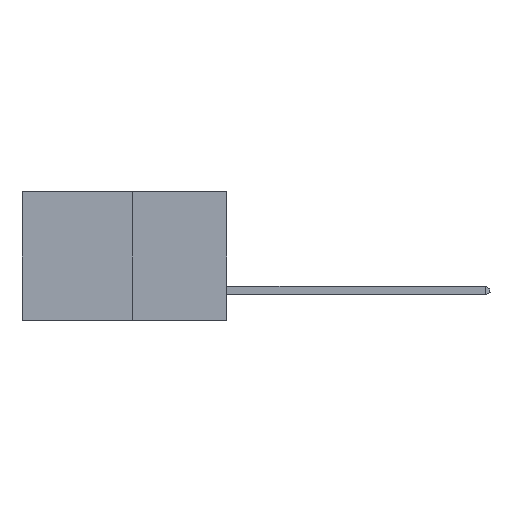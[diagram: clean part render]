
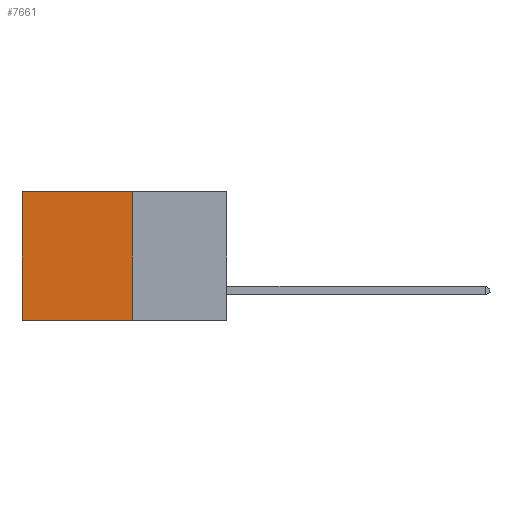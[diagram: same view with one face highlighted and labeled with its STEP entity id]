
A CAD part, left-side view. The second image highlights one B-rep face of the part: STEP entity #7661.
In plain terms, the highlighted planar face has unit normal (-1, 0, 0).
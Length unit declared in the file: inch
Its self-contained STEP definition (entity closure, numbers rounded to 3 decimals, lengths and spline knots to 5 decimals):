
#938 = EDGE_LOOP ( 'NONE', ( #30658, #7178, #3249, #1567 ) ) ;
#1088 = VERTEX_POINT ( 'NONE', #22789 ) ;
#1567 = ORIENTED_EDGE ( 'NONE', *, *, #18640, .T. ) ;
#1786 = DIRECTION ( 'NONE',  ( 0., 0., -1. ) ) ;
#2138 = DIRECTION ( 'NONE',  ( 0., 1., 0. ) ) ;
#2320 = DIRECTION ( 'NONE',  ( 0., 0., -1. ) ) ;
#3249 = ORIENTED_EDGE ( 'NONE', *, *, #10928, .F. ) ;
#3741 = CARTESIAN_POINT ( 'NONE',  ( 0.277, 0.27, -0.37 ) ) ;
#3883 = DIRECTION ( 'NONE',  ( 1., 0., 0. ) ) ;
#7178 = ORIENTED_EDGE ( 'NONE', *, *, #29767, .F. ) ;
#7661 = ADVANCED_FACE ( 'NONE', ( #13336 ), #24814, .F. ) ;
#8039 = CARTESIAN_POINT ( 'NONE',  ( 0.277, 0.59, 0. ) ) ;
#10627 = VERTEX_POINT ( 'NONE', #16747 ) ;
#10928 = EDGE_CURVE ( 'NONE', #10627, #14963, #24257, .T. ) ;
#13336 = FACE_OUTER_BOUND ( 'NONE', #938, .T. ) ;
#14853 = VECTOR ( 'NONE', #2138, 39.37008 ) ;
#14963 = VERTEX_POINT ( 'NONE', #3741 ) ;
#15121 = AXIS2_PLACEMENT_3D ( 'NONE', #19726, #3883, #22331 ) ;
#16747 = CARTESIAN_POINT ( 'NONE',  ( 0.277, 0.27, 0. ) ) ;
#17963 = CARTESIAN_POINT ( 'NONE',  ( 0.277, 0.27, -0.37 ) ) ;
#18640 = EDGE_CURVE ( 'NONE', #10627, #21871, #26075, .T. ) ;
#18955 = VECTOR ( 'NONE', #2320, 39.37008 ) ;
#19156 = VECTOR ( 'NONE', #22991, 39.37008 ) ;
#19726 = CARTESIAN_POINT ( 'NONE',  ( 0.277, 0.27, -0.37 ) ) ;
#20398 = CARTESIAN_POINT ( 'NONE',  ( 0.277, 0.27, -0.37 ) ) ;
#21871 = VERTEX_POINT ( 'NONE', #8039 ) ;
#22331 = DIRECTION ( 'NONE',  ( 0., 0., -1. ) ) ;
#22789 = CARTESIAN_POINT ( 'NONE',  ( 0.277, 0.59, -0.37 ) ) ;
#22866 = EDGE_CURVE ( 'NONE', #21871, #1088, #32841, .T. ) ;
#22881 = CARTESIAN_POINT ( 'NONE',  ( 0.277, 0.27, 0. ) ) ;
#22991 = DIRECTION ( 'NONE',  ( 0., 1., 0. ) ) ;
#24257 = LINE ( 'NONE', #20398, #25059 ) ;
#24814 = PLANE ( 'NONE',  #15121 ) ;
#25059 = VECTOR ( 'NONE', #1786, 39.37008 ) ;
#26075 = LINE ( 'NONE', #22881, #19156 ) ;
#29558 = LINE ( 'NONE', #17963, #14853 ) ;
#29767 = EDGE_CURVE ( 'NONE', #14963, #1088, #29558, .T. ) ;
#30658 = ORIENTED_EDGE ( 'NONE', *, *, #22866, .T. ) ;
#32841 = LINE ( 'NONE', #33941, #18955 ) ;
#33941 = CARTESIAN_POINT ( 'NONE',  ( 0.277, 0.59, -0.37 ) ) ;
